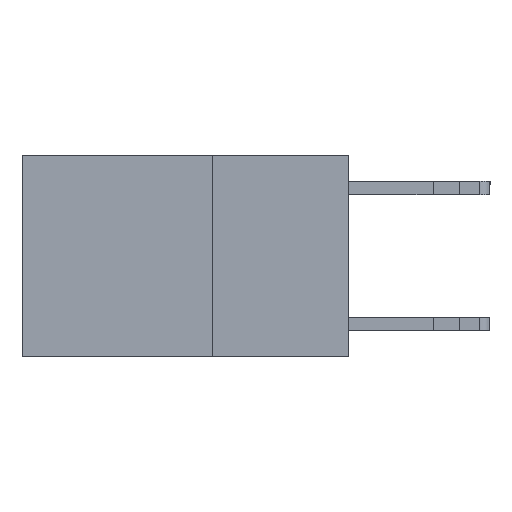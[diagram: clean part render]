
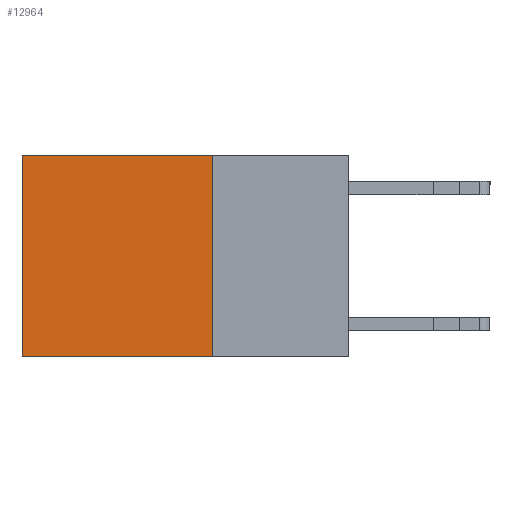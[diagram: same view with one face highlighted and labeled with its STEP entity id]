
A CAD part, left-side view. The second image highlights one B-rep face of the part: STEP entity #12964.
In plain terms, the highlighted planar face has unit normal (-1, 0, 0).
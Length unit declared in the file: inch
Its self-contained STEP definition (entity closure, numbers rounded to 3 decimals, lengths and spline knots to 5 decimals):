
#949 = DIRECTION ( 'NONE',  ( 0., 1., 0. ) ) ;
#1110 = CARTESIAN_POINT ( 'NONE',  ( 0.2625, 0.25, -0.37 ) ) ;
#1129 = VERTEX_POINT ( 'NONE', #6112 ) ;
#1374 = ORIENTED_EDGE ( 'NONE', *, *, #6717, .T. ) ;
#1732 = DIRECTION ( 'NONE',  ( 0., 0., -1. ) ) ;
#2397 = DIRECTION ( 'NONE',  ( 1., 0., 0. ) ) ;
#2786 = CARTESIAN_POINT ( 'NONE',  ( 0.2625, 0.6, 0. ) ) ;
#3060 = VECTOR ( 'NONE', #1732, 39.37008 ) ;
#3459 = LINE ( 'NONE', #1110, #12771 ) ;
#3499 = DIRECTION ( 'NONE',  ( 0., 0., -1. ) ) ;
#3573 = CARTESIAN_POINT ( 'NONE',  ( 0.2625, 0.25, 0. ) ) ;
#3600 = FACE_OUTER_BOUND ( 'NONE', #13924, .T. ) ;
#3860 = EDGE_CURVE ( 'NONE', #10213, #1129, #14539, .T. ) ;
#5081 = CARTESIAN_POINT ( 'NONE',  ( 0.2625, 0.25, 0. ) ) ;
#5665 = EDGE_CURVE ( 'NONE', #10213, #8046, #15065, .T. ) ;
#5990 = AXIS2_PLACEMENT_3D ( 'NONE', #11115, #2397, #6342 ) ;
#6112 = CARTESIAN_POINT ( 'NONE',  ( 0.2625, 0.25, -0.37 ) ) ;
#6342 = DIRECTION ( 'NONE',  ( 0., 0., -1. ) ) ;
#6413 = ORIENTED_EDGE ( 'NONE', *, *, #5665, .T. ) ;
#6717 = EDGE_CURVE ( 'NONE', #8046, #9427, #7903, .T. ) ;
#7092 = CARTESIAN_POINT ( 'NONE',  ( 0.2625, 0.6, -0.37 ) ) ;
#7903 = LINE ( 'NONE', #2786, #3060 ) ;
#8046 = VERTEX_POINT ( 'NONE', #11648 ) ;
#8578 = PLANE ( 'NONE',  #5990 ) ;
#8973 = VECTOR ( 'NONE', #13690, 39.37008 ) ;
#9059 = EDGE_CURVE ( 'NONE', #1129, #9427, #3459, .T. ) ;
#9427 = VERTEX_POINT ( 'NONE', #7092 ) ;
#9716 = VECTOR ( 'NONE', #3499, 39.37008 ) ;
#10213 = VERTEX_POINT ( 'NONE', #11781 ) ;
#11115 = CARTESIAN_POINT ( 'NONE',  ( 0.2625, 0.25, 0. ) ) ;
#11648 = CARTESIAN_POINT ( 'NONE',  ( 0.2625, 0.6, 0. ) ) ;
#11781 = CARTESIAN_POINT ( 'NONE',  ( 0.2625, 0.25, 0. ) ) ;
#12771 = VECTOR ( 'NONE', #949, 39.37008 ) ;
#12964 = ADVANCED_FACE ( 'NONE', ( #3600 ), #8578, .F. ) ;
#13690 = DIRECTION ( 'NONE',  ( 0., 1., 0. ) ) ;
#13924 = EDGE_LOOP ( 'NONE', ( #1374, #13993, #14225, #6413 ) ) ;
#13993 = ORIENTED_EDGE ( 'NONE', *, *, #9059, .F. ) ;
#14225 = ORIENTED_EDGE ( 'NONE', *, *, #3860, .F. ) ;
#14539 = LINE ( 'NONE', #3573, #9716 ) ;
#15065 = LINE ( 'NONE', #5081, #8973 ) ;
